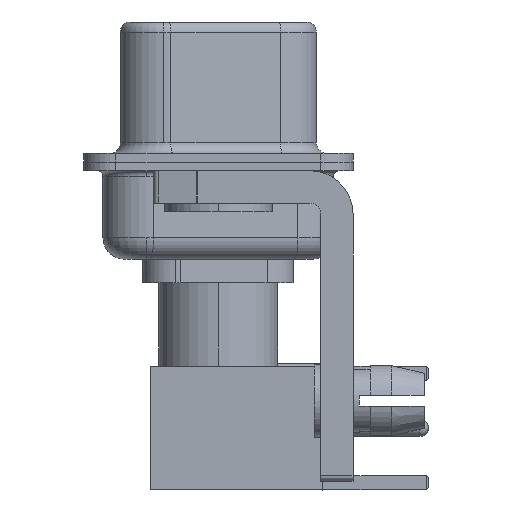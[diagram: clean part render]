
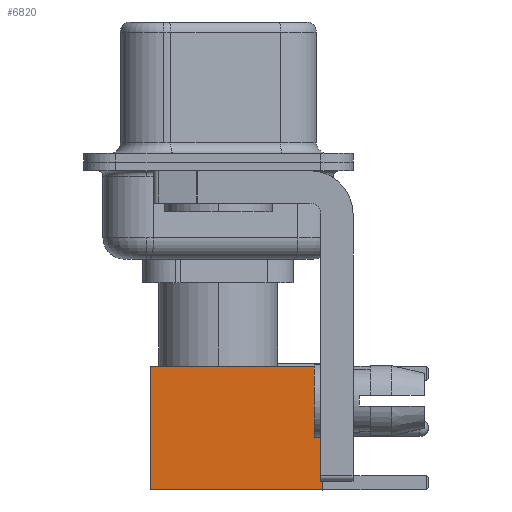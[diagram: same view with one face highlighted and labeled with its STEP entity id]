
A CAD part, left-side view. The second image highlights one B-rep face of the part: STEP entity #6820.
In plain terms, the highlighted face is planar.
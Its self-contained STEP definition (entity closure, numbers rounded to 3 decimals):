
#1442 = DIRECTION ( 'NONE',  ( 0., 0., -1. ) ) ;
#2188 = PLANE ( 'NONE',  #24976 ) ;
#2464 = ORIENTED_EDGE ( 'NONE', *, *, #26232, .T. ) ;
#4492 = CARTESIAN_POINT ( 'NONE',  ( 2.875, 2.875, 0. ) ) ;
#4634 = VERTEX_POINT ( 'NONE', #10762 ) ;
#5118 = DIRECTION ( 'NONE',  ( 0., 0., -1. ) ) ;
#6138 = VERTEX_POINT ( 'NONE', #15088 ) ;
#6820 = ADVANCED_FACE ( 'NONE', ( #9420 ), #2188, .T. ) ;
#7365 = ORIENTED_EDGE ( 'NONE', *, *, #13535, .F. ) ;
#8197 = EDGE_LOOP ( 'NONE', ( #16233, #2464, #16672, #7365 ) ) ;
#8378 = VERTEX_POINT ( 'NONE', #22444 ) ;
#8688 = CARTESIAN_POINT ( 'NONE',  ( -2.875, 2.875, 0. ) ) ;
#9420 = FACE_OUTER_BOUND ( 'NONE', #8197, .T. ) ;
#10762 = CARTESIAN_POINT ( 'NONE',  ( -2.875, 2.875, 8. ) ) ;
#10995 = VECTOR ( 'NONE', #5118, 1000. ) ;
#12495 = CARTESIAN_POINT ( 'NONE',  ( 0., 2.875, 8. ) ) ;
#12976 = VECTOR ( 'NONE', #1442, 1000. ) ;
#13355 = LINE ( 'NONE', #8688, #12976 ) ;
#13535 = EDGE_CURVE ( 'NONE', #16850, #4634, #19933, .T. ) ;
#14765 = VECTOR ( 'NONE', #17751, 1000. ) ;
#14881 = LINE ( 'NONE', #22176, #18174 ) ;
#15088 = CARTESIAN_POINT ( 'NONE',  ( 2.875, 2.875, 0. ) ) ;
#16233 = ORIENTED_EDGE ( 'NONE', *, *, #20314, .T. ) ;
#16672 = ORIENTED_EDGE ( 'NONE', *, *, #19997, .F. ) ;
#16850 = VERTEX_POINT ( 'NONE', #23868 ) ;
#17751 = DIRECTION ( 'NONE',  ( -1., 0., 0. ) ) ;
#18174 = VECTOR ( 'NONE', #19838, 1000. ) ;
#19838 = DIRECTION ( 'NONE',  ( -1., 0., 0. ) ) ;
#19933 = LINE ( 'NONE', #12495, #14765 ) ;
#19997 = EDGE_CURVE ( 'NONE', #4634, #8378, #13355, .T. ) ;
#20314 = EDGE_CURVE ( 'NONE', #16850, #6138, #28638, .T. ) ;
#22176 = CARTESIAN_POINT ( 'NONE',  ( 0., 2.875, 0. ) ) ;
#22444 = CARTESIAN_POINT ( 'NONE',  ( -2.875, 2.875, 0. ) ) ;
#23868 = CARTESIAN_POINT ( 'NONE',  ( 2.875, 2.875, 8. ) ) ;
#24976 = AXIS2_PLACEMENT_3D ( 'NONE', #4492, #30483, #25849 ) ;
#25849 = DIRECTION ( 'NONE',  ( 0., 0., 1. ) ) ;
#26232 = EDGE_CURVE ( 'NONE', #6138, #8378, #14881, .T. ) ;
#26318 = CARTESIAN_POINT ( 'NONE',  ( 2.875, 2.875, 0. ) ) ;
#28638 = LINE ( 'NONE', #26318, #10995 ) ;
#30483 = DIRECTION ( 'NONE',  ( 0., 1., 0. ) ) ;
